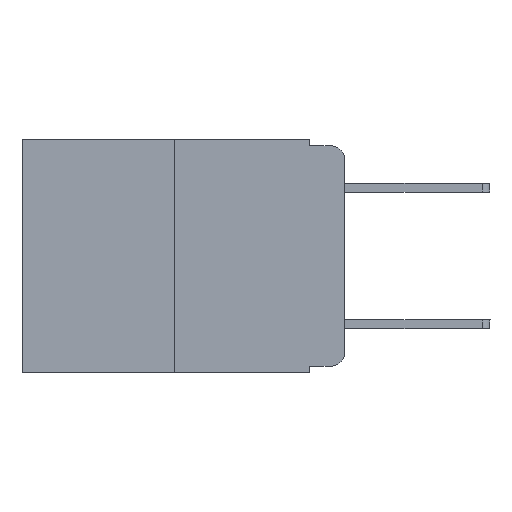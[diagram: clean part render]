
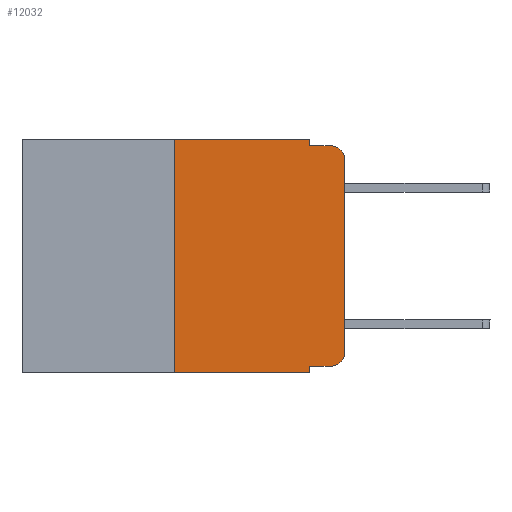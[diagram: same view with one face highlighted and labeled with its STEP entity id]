
A CAD part, left-side view. The second image highlights one B-rep face of the part: STEP entity #12032.
In plain terms, the highlighted planar face has unit normal (-1, 0, 0).
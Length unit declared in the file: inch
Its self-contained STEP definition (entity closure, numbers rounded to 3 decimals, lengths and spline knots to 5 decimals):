
#6 = DIRECTION ( 'NONE',  ( 0., -1., 0. ) ) ;
#181 = EDGE_CURVE ( 'NONE', #6424, #10267, #6490, .T. ) ;
#253 = VERTEX_POINT ( 'NONE', #10050 ) ;
#377 = CARTESIAN_POINT ( 'NONE',  ( 0., 0.473, 0. ) ) ;
#438 = VECTOR ( 'NONE', #2188, 39.37008 ) ;
#776 = CARTESIAN_POINT ( 'NONE',  ( 0., 0.473, 0. ) ) ;
#896 = VECTOR ( 'NONE', #7946, 39.37008 ) ;
#958 = DIRECTION ( 'NONE',  ( 0., 0., -1. ) ) ;
#1050 = DIRECTION ( 'NONE',  ( -1., 0., 0. ) ) ;
#1723 = CARTESIAN_POINT ( 'NONE',  ( 0., 0.25, -0.343 ) ) ;
#1981 = FACE_OUTER_BOUND ( 'NONE', #3612, .T. ) ;
#1994 = EDGE_CURVE ( 'NONE', #253, #5884, #5929, .T. ) ;
#2168 = CARTESIAN_POINT ( 'NONE',  ( 0., 0.02, -0.313 ) ) ;
#2178 = VECTOR ( 'NONE', #9690, 39.37008 ) ;
#2188 = DIRECTION ( 'NONE',  ( 0., 0., 1. ) ) ;
#2367 = CARTESIAN_POINT ( 'NONE',  ( 0., 0.051, -0.343 ) ) ;
#2576 = CARTESIAN_POINT ( 'NONE',  ( 0., 0.051, -0.01 ) ) ;
#3018 = CARTESIAN_POINT ( 'NONE',  ( 0., 0., -0.03 ) ) ;
#3612 = EDGE_LOOP ( 'NONE', ( #4376, #11619, #4616, #11607, #12794, #11597, #5453, #6269, #13546, #12080 ) ) ;
#3631 = CARTESIAN_POINT ( 'NONE',  ( 0., 0.051, -0.01 ) ) ;
#3639 = VECTOR ( 'NONE', #10163, 39.37008 ) ;
#3846 = VERTEX_POINT ( 'NONE', #10736 ) ;
#4005 = AXIS2_PLACEMENT_3D ( 'NONE', #776, #12607, #11640 ) ;
#4038 = EDGE_CURVE ( 'NONE', #11287, #6424, #8052, .T. ) ;
#4326 = EDGE_CURVE ( 'NONE', #5884, #3846, #12630, .T. ) ;
#4340 = CARTESIAN_POINT ( 'NONE',  ( 0., 0.051, -0.333 ) ) ;
#4376 = ORIENTED_EDGE ( 'NONE', *, *, #181, .T. ) ;
#4616 = ORIENTED_EDGE ( 'NONE', *, *, #4326, .F. ) ;
#4644 = EDGE_CURVE ( 'NONE', #11485, #7558, #7355, .T. ) ;
#4717 = VECTOR ( 'NONE', #6, 39.37008 ) ;
#5002 = PLANE ( 'NONE',  #4005 ) ;
#5453 = ORIENTED_EDGE ( 'NONE', *, *, #11664, .T. ) ;
#5884 = VERTEX_POINT ( 'NONE', #3631 ) ;
#5929 = LINE ( 'NONE', #5959, #896 ) ;
#5959 = CARTESIAN_POINT ( 'NONE',  ( 0., 0.051, 0. ) ) ;
#6015 = VECTOR ( 'NONE', #11246, 39.37008 ) ;
#6269 = ORIENTED_EDGE ( 'NONE', *, *, #11118, .F. ) ;
#6424 = VERTEX_POINT ( 'NONE', #9980 ) ;
#6490 = LINE ( 'NONE', #13072, #438 ) ;
#6705 = LINE ( 'NONE', #12793, #9734 ) ;
#6833 = VERTEX_POINT ( 'NONE', #4340 ) ;
#7041 = CARTESIAN_POINT ( 'NONE',  ( 0., 0.25, 0. ) ) ;
#7300 = LINE ( 'NONE', #9614, #4717 ) ;
#7355 = LINE ( 'NONE', #7041, #6015 ) ;
#7558 = VERTEX_POINT ( 'NONE', #9860 ) ;
#7900 = DIRECTION ( 'NONE',  ( 0., -1., 0. ) ) ;
#7946 = DIRECTION ( 'NONE',  ( 0., 0., -1. ) ) ;
#7972 = VERTEX_POINT ( 'NONE', #2367 ) ;
#8052 = CIRCLE ( 'NONE', #11392, 0.02 ) ;
#8097 = VECTOR ( 'NONE', #7900, 39.37008 ) ;
#8422 = EDGE_CURVE ( 'NONE', #6833, #11287, #7300, .T. ) ;
#9253 = CIRCLE ( 'NONE', #11436, 0.02 ) ;
#9516 = DIRECTION ( 'NONE',  ( 0., 0., -1. ) ) ;
#9540 = EDGE_CURVE ( 'NONE', #7558, #253, #11999, .T. ) ;
#9588 = CARTESIAN_POINT ( 'NONE',  ( 0., 0.02, -0.03 ) ) ;
#9614 = CARTESIAN_POINT ( 'NONE',  ( 0., 0.051, -0.333 ) ) ;
#9690 = DIRECTION ( 'NONE',  ( 0., 0., -1. ) ) ;
#9734 = VECTOR ( 'NONE', #10773, 39.37008 ) ;
#9789 = EDGE_CURVE ( 'NONE', #10267, #3846, #9253, .T. ) ;
#9860 = CARTESIAN_POINT ( 'NONE',  ( 0., 0.25, 0. ) ) ;
#9980 = CARTESIAN_POINT ( 'NONE',  ( 0., 0., -0.313 ) ) ;
#10050 = CARTESIAN_POINT ( 'NONE',  ( 0., 0.051, 0. ) ) ;
#10163 = DIRECTION ( 'NONE',  ( 0., -1., 0. ) ) ;
#10267 = VERTEX_POINT ( 'NONE', #3018 ) ;
#10736 = CARTESIAN_POINT ( 'NONE',  ( 0., 0.02, -0.01 ) ) ;
#10773 = DIRECTION ( 'NONE',  ( 0., -1., 0. ) ) ;
#10789 = LINE ( 'NONE', #10834, #2178 ) ;
#10834 = CARTESIAN_POINT ( 'NONE',  ( 0., 0.051, 0. ) ) ;
#11118 = EDGE_CURVE ( 'NONE', #6833, #7972, #10789, .T. ) ;
#11246 = DIRECTION ( 'NONE',  ( 0., 0., 1. ) ) ;
#11287 = VERTEX_POINT ( 'NONE', #13231 ) ;
#11392 = AXIS2_PLACEMENT_3D ( 'NONE', #2168, #12818, #9516 ) ;
#11436 = AXIS2_PLACEMENT_3D ( 'NONE', #9588, #1050, #958 ) ;
#11485 = VERTEX_POINT ( 'NONE', #1723 ) ;
#11597 = ORIENTED_EDGE ( 'NONE', *, *, #4644, .F. ) ;
#11607 = ORIENTED_EDGE ( 'NONE', *, *, #1994, .F. ) ;
#11619 = ORIENTED_EDGE ( 'NONE', *, *, #9789, .T. ) ;
#11640 = DIRECTION ( 'NONE',  ( 0., 0., -1. ) ) ;
#11664 = EDGE_CURVE ( 'NONE', #11485, #7972, #6705, .T. ) ;
#11999 = LINE ( 'NONE', #377, #8097 ) ;
#12032 = ADVANCED_FACE ( 'NONE', ( #1981 ), #5002, .F. ) ;
#12080 = ORIENTED_EDGE ( 'NONE', *, *, #4038, .T. ) ;
#12607 = DIRECTION ( 'NONE',  ( 1., 0., 0. ) ) ;
#12630 = LINE ( 'NONE', #2576, #3639 ) ;
#12793 = CARTESIAN_POINT ( 'NONE',  ( 0., 0.473, -0.343 ) ) ;
#12794 = ORIENTED_EDGE ( 'NONE', *, *, #9540, .F. ) ;
#12818 = DIRECTION ( 'NONE',  ( -1., 0., 0. ) ) ;
#13072 = CARTESIAN_POINT ( 'NONE',  ( 0., 0., 0. ) ) ;
#13231 = CARTESIAN_POINT ( 'NONE',  ( 0., 0.02, -0.333 ) ) ;
#13546 = ORIENTED_EDGE ( 'NONE', *, *, #8422, .T. ) ;
